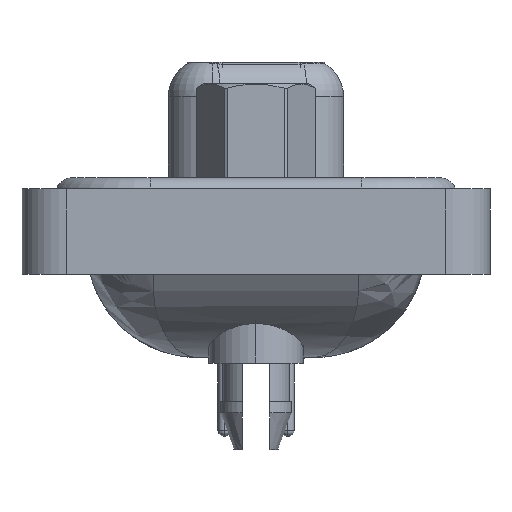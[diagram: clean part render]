
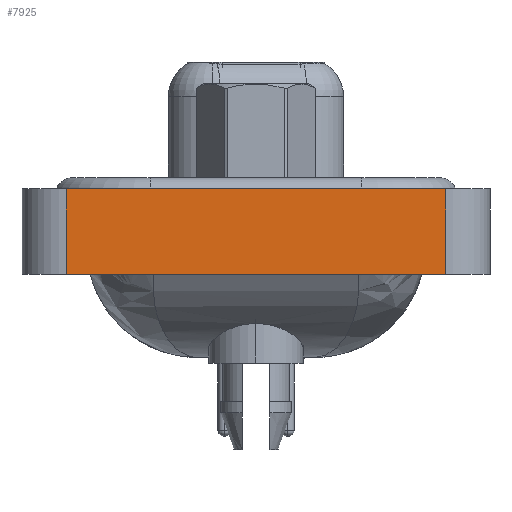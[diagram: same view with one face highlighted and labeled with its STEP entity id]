
A CAD part, left-side view. The second image highlights one B-rep face of the part: STEP entity #7925.
In plain terms, the highlighted planar face has unit normal (-1, 0, 0).
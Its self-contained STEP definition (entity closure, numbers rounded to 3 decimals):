
#1100 = DIRECTION ( 'NONE',  ( 0., 0., 1. ) ) ;
#1615 = LINE ( 'NONE', #17859, #14877 ) ;
#2064 = LINE ( 'NONE', #11230, #12075 ) ;
#3404 = AXIS2_PLACEMENT_3D ( 'NONE', #22473, #11040, #10748 ) ;
#5770 = LINE ( 'NONE', #21714, #20910 ) ;
#6244 = FACE_OUTER_BOUND ( 'NONE', #11763, .T. ) ;
#6633 = ORIENTED_EDGE ( 'NONE', *, *, #25427, .F. ) ;
#6827 = DIRECTION ( 'NONE',  ( 0., -1., 0. ) ) ;
#7925 = ADVANCED_FACE ( 'NONE', ( #6244 ), #13309, .T. ) ;
#8001 = VERTEX_POINT ( 'NONE', #15559 ) ;
#8733 = ORIENTED_EDGE ( 'NONE', *, *, #24864, .F. ) ;
#10748 = DIRECTION ( 'NONE',  ( 0., 0., 1. ) ) ;
#11040 = DIRECTION ( 'NONE',  ( -1., 0., 0. ) ) ;
#11230 = CARTESIAN_POINT ( 'NONE',  ( -7.225, -8.55, -3.35 ) ) ;
#11763 = EDGE_LOOP ( 'NONE', ( #24411, #6633, #8733, #20177 ) ) ;
#12075 = VECTOR ( 'NONE', #20405, 1000. ) ;
#13309 = PLANE ( 'NONE',  #3404 ) ;
#13365 = CARTESIAN_POINT ( 'NONE',  ( -7.225, -8.55, 0.5 ) ) ;
#14424 = EDGE_CURVE ( 'NONE', #14720, #8001, #2064, .T. ) ;
#14720 = VERTEX_POINT ( 'NONE', #26084 ) ;
#14877 = VECTOR ( 'NONE', #26711, 1000. ) ;
#15287 = EDGE_CURVE ( 'NONE', #8001, #21325, #5770, .T. ) ;
#15559 = CARTESIAN_POINT ( 'NONE',  ( -7.225, -8.55, -3.35 ) ) ;
#17859 = CARTESIAN_POINT ( 'NONE',  ( -7.225, 8.55, -3.35 ) ) ;
#18249 = LINE ( 'NONE', #29652, #24037 ) ;
#20177 = ORIENTED_EDGE ( 'NONE', *, *, #14424, .T. ) ;
#20405 = DIRECTION ( 'NONE',  ( 0., -1., 0. ) ) ;
#20910 = VECTOR ( 'NONE', #1100, 1000. ) ;
#21325 = VERTEX_POINT ( 'NONE', #13365 ) ;
#21714 = CARTESIAN_POINT ( 'NONE',  ( -7.225, -8.55, -3.35 ) ) ;
#22473 = CARTESIAN_POINT ( 'NONE',  ( -7.225, -8.55, -3.35 ) ) ;
#24037 = VECTOR ( 'NONE', #6827, 1000. ) ;
#24411 = ORIENTED_EDGE ( 'NONE', *, *, #15287, .T. ) ;
#24864 = EDGE_CURVE ( 'NONE', #14720, #29133, #1615, .T. ) ;
#25427 = EDGE_CURVE ( 'NONE', #29133, #21325, #18249, .T. ) ;
#26084 = CARTESIAN_POINT ( 'NONE',  ( -7.225, 8.55, -3.35 ) ) ;
#26711 = DIRECTION ( 'NONE',  ( 0., 0., 1. ) ) ;
#28460 = CARTESIAN_POINT ( 'NONE',  ( -7.225, 8.55, 0.5 ) ) ;
#29133 = VERTEX_POINT ( 'NONE', #28460 ) ;
#29652 = CARTESIAN_POINT ( 'NONE',  ( -7.225, -8.55, 0.5 ) ) ;
